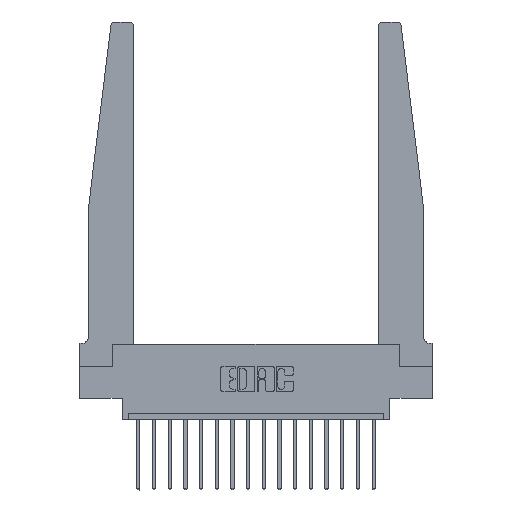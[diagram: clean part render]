
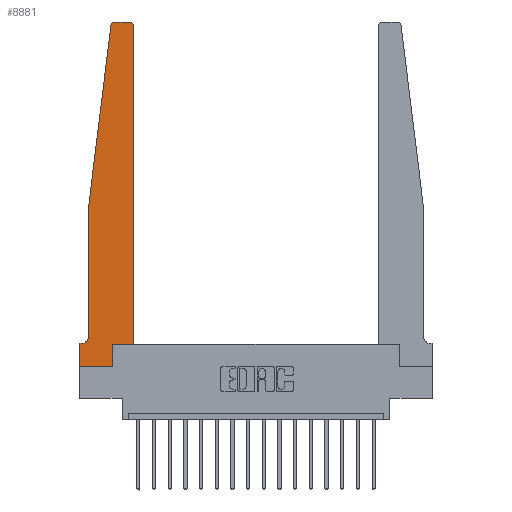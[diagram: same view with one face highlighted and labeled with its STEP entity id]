
A CAD part, top view. The second image highlights one B-rep face of the part: STEP entity #8881.
In plain terms, the highlighted planar face has unit normal (0, 0, 1).
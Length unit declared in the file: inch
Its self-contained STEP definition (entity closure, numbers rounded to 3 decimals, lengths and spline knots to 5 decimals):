
#264 = DIRECTION ( 'NONE',  ( 1., 0., 0. ) ) ;
#283 = ORIENTED_EDGE ( 'NONE', *, *, #673, .T. ) ;
#622 = VERTEX_POINT ( 'NONE', #10857 ) ;
#643 = ORIENTED_EDGE ( 'NONE', *, *, #16864, .T. ) ;
#673 = EDGE_CURVE ( 'NONE', #8094, #17624, #799, .T. ) ;
#678 = ORIENTED_EDGE ( 'NONE', *, *, #14384, .T. ) ;
#799 = LINE ( 'NONE', #3755, #14377 ) ;
#1018 = VERTEX_POINT ( 'NONE', #7943 ) ;
#1163 = EDGE_CURVE ( 'NONE', #3932, #12456, #2162, .T. ) ;
#1509 = CARTESIAN_POINT ( 'NONE',  ( 0.015, 0.1875, 0.37 ) ) ;
#1540 = DIRECTION ( 'NONE',  ( 0., 0., 1. ) ) ;
#1717 = CARTESIAN_POINT ( 'NONE',  ( 0., 0., 0.37 ) ) ;
#1989 = LINE ( 'NONE', #9627, #13992 ) ;
#2085 = CARTESIAN_POINT ( 'NONE',  ( 0.015, 0.2375, 0.37 ) ) ;
#2162 = LINE ( 'NONE', #2387, #3278 ) ;
#2244 = VERTEX_POINT ( 'NONE', #3227 ) ;
#2333 = ORIENTED_EDGE ( 'NONE', *, *, #7165, .T. ) ;
#2387 = CARTESIAN_POINT ( 'NONE',  ( 0., 0., 0.37 ) ) ;
#2497 = FACE_OUTER_BOUND ( 'NONE', #12037, .T. ) ;
#3054 = VECTOR ( 'NONE', #264, 39.37008 ) ;
#3227 = CARTESIAN_POINT ( 'NONE',  ( 0.395, 2.75, 0.37 ) ) ;
#3278 = VECTOR ( 'NONE', #12420, 39.37008 ) ;
#3329 = EDGE_CURVE ( 'NONE', #10567, #1018, #18221, .T. ) ;
#3332 = DIRECTION ( 'NONE',  ( 0., 1., 0. ) ) ;
#3462 = DIRECTION ( 'NONE',  ( 0., 0., -1. ) ) ;
#3755 = CARTESIAN_POINT ( 'NONE',  ( 0.065, 1.25, 0.37 ) ) ;
#3794 = ORIENTED_EDGE ( 'NONE', *, *, #3329, .T. ) ;
#3932 = VERTEX_POINT ( 'NONE', #3984 ) ;
#3984 = CARTESIAN_POINT ( 'NONE',  ( 0., 0.1875, 0.37 ) ) ;
#4207 = CARTESIAN_POINT ( 'NONE',  ( 0.27653, 2.72, 0.37 ) ) ;
#4395 = DIRECTION ( 'NONE',  ( 1., 0., 0. ) ) ;
#4505 = AXIS2_PLACEMENT_3D ( 'NONE', #4207, #5679, #18316 ) ;
#4579 = LINE ( 'NONE', #4690, #17170 ) ;
#4690 = CARTESIAN_POINT ( 'NONE',  ( 0.2605, 0.18, 0.37 ) ) ;
#5086 = VERTEX_POINT ( 'NONE', #17884 ) ;
#5114 = LINE ( 'NONE', #11923, #17284 ) ;
#5201 = EDGE_CURVE ( 'NONE', #1018, #5086, #1989, .T. ) ;
#5377 = EDGE_CURVE ( 'NONE', #15715, #3932, #10888, .T. ) ;
#5427 = AXIS2_PLACEMENT_3D ( 'NONE', #2085, #3462, #6120 ) ;
#5679 = DIRECTION ( 'NONE',  ( 0., 0., 1. ) ) ;
#5896 = DIRECTION ( 'NONE',  ( 1., 0., 0. ) ) ;
#6120 = DIRECTION ( 'NONE',  ( -1., 0., 0. ) ) ;
#6558 = DIRECTION ( 'NONE',  ( 0., -1., 0. ) ) ;
#6586 = ORIENTED_EDGE ( 'NONE', *, *, #13742, .T. ) ;
#6753 = DIRECTION ( 'NONE',  ( -1., 0., 0. ) ) ;
#7105 = VECTOR ( 'NONE', #15239, 39.37008 ) ;
#7147 = CARTESIAN_POINT ( 'NONE',  ( 0.425, 0.18, 0.37 ) ) ;
#7165 = EDGE_CURVE ( 'NONE', #622, #10567, #4579, .T. ) ;
#7317 = CIRCLE ( 'NONE', #5427, 0.05 ) ;
#7412 = CARTESIAN_POINT ( 'NONE',  ( 0., 0.1875, 0.37 ) ) ;
#7943 = CARTESIAN_POINT ( 'NONE',  ( 0.425, 0.18, 0.37 ) ) ;
#8094 = VERTEX_POINT ( 'NONE', #17527 ) ;
#8126 = CARTESIAN_POINT ( 'NONE',  ( 0.24675, 2.72367, 0.37 ) ) ;
#8327 = VERTEX_POINT ( 'NONE', #8126 ) ;
#8543 = CARTESIAN_POINT ( 'NONE',  ( 0.2605, 0.18, 0.37 ) ) ;
#8791 = LINE ( 'NONE', #15118, #10315 ) ;
#8881 = ADVANCED_FACE ( 'NONE', ( #2497 ), #8909, .T. ) ;
#8909 = PLANE ( 'NONE',  #10383 ) ;
#9244 = ORIENTED_EDGE ( 'NONE', *, *, #5377, .T. ) ;
#9627 = CARTESIAN_POINT ( 'NONE',  ( 0.425, 0.18, 0.37 ) ) ;
#9972 = ORIENTED_EDGE ( 'NONE', *, *, #10100, .T. ) ;
#10080 = DIRECTION ( 'NONE',  ( 0., 0., 1. ) ) ;
#10100 = EDGE_CURVE ( 'NONE', #8327, #8094, #5114, .T. ) ;
#10107 = CARTESIAN_POINT ( 'NONE',  ( 0., 0., 0.37 ) ) ;
#10136 = DIRECTION ( 'NONE',  ( 1., 0., 0. ) ) ;
#10315 = VECTOR ( 'NONE', #6753, 39.37008 ) ;
#10383 = AXIS2_PLACEMENT_3D ( 'NONE', #7412, #10080, #10136 ) ;
#10567 = VERTEX_POINT ( 'NONE', #8543 ) ;
#10578 = EDGE_CURVE ( 'NONE', #5086, #2244, #14184, .T. ) ;
#10579 = LINE ( 'NONE', #1717, #3054 ) ;
#10857 = CARTESIAN_POINT ( 'NONE',  ( 0.2605, 0., 0.37 ) ) ;
#10888 = LINE ( 'NONE', #16831, #7105 ) ;
#10945 = EDGE_CURVE ( 'NONE', #17624, #15715, #7317, .T. ) ;
#11179 = VECTOR ( 'NONE', #4395, 39.37008 ) ;
#11592 = CARTESIAN_POINT ( 'NONE',  ( 0.395, 2.72, 0.37 ) ) ;
#11923 = CARTESIAN_POINT ( 'NONE',  ( 0.065, 1.25, 0.37 ) ) ;
#12037 = EDGE_LOOP ( 'NONE', ( #678, #643, #9972, #283, #17844, #9244, #12538, #6586, #2333, #3794, #13257, #14338 ) ) ;
#12420 = DIRECTION ( 'NONE',  ( 0., -1., 0. ) ) ;
#12456 = VERTEX_POINT ( 'NONE', #10107 ) ;
#12538 = ORIENTED_EDGE ( 'NONE', *, *, #1163, .T. ) ;
#13257 = ORIENTED_EDGE ( 'NONE', *, *, #5201, .T. ) ;
#13742 = EDGE_CURVE ( 'NONE', #12456, #622, #10579, .T. ) ;
#13992 = VECTOR ( 'NONE', #16747, 39.37008 ) ;
#14184 = CIRCLE ( 'NONE', #17487, 0.03 ) ;
#14338 = ORIENTED_EDGE ( 'NONE', *, *, #10578, .T. ) ;
#14377 = VECTOR ( 'NONE', #6558, 39.37008 ) ;
#14384 = EDGE_CURVE ( 'NONE', #2244, #14484, #8791, .T. ) ;
#14484 = VERTEX_POINT ( 'NONE', #18234 ) ;
#15118 = CARTESIAN_POINT ( 'NONE',  ( 0.25, 2.75, 0.37 ) ) ;
#15239 = DIRECTION ( 'NONE',  ( -1., 0., 0. ) ) ;
#15715 = VERTEX_POINT ( 'NONE', #1509 ) ;
#16747 = DIRECTION ( 'NONE',  ( 0., 1., 0. ) ) ;
#16831 = CARTESIAN_POINT ( 'NONE',  ( 0.065, 0.1875, 0.37 ) ) ;
#16864 = EDGE_CURVE ( 'NONE', #14484, #8327, #17539, .T. ) ;
#17026 = DIRECTION ( 'NONE',  ( -0.122, -0.992, 0. ) ) ;
#17170 = VECTOR ( 'NONE', #3332, 39.37008 ) ;
#17284 = VECTOR ( 'NONE', #17026, 39.37008 ) ;
#17487 = AXIS2_PLACEMENT_3D ( 'NONE', #11592, #1540, #5896 ) ;
#17527 = CARTESIAN_POINT ( 'NONE',  ( 0.065, 1.25, 0.37 ) ) ;
#17539 = CIRCLE ( 'NONE', #4505, 0.03 ) ;
#17624 = VERTEX_POINT ( 'NONE', #18039 ) ;
#17844 = ORIENTED_EDGE ( 'NONE', *, *, #10945, .T. ) ;
#17884 = CARTESIAN_POINT ( 'NONE',  ( 0.425, 2.72, 0.37 ) ) ;
#18039 = CARTESIAN_POINT ( 'NONE',  ( 0.065, 0.2375, 0.37 ) ) ;
#18221 = LINE ( 'NONE', #7147, #11179 ) ;
#18234 = CARTESIAN_POINT ( 'NONE',  ( 0.27653, 2.75, 0.37 ) ) ;
#18316 = DIRECTION ( 'NONE',  ( 1., 0., 0. ) ) ;
